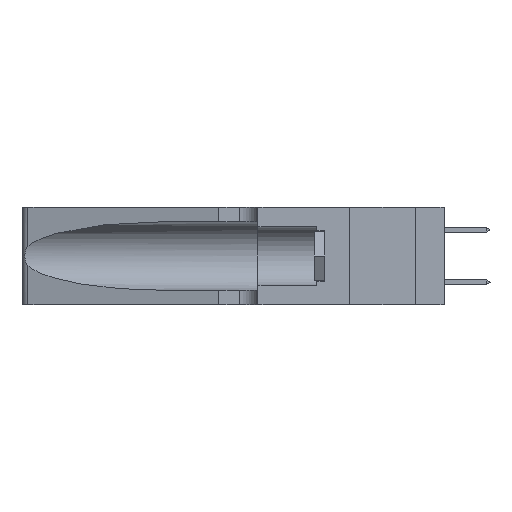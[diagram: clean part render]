
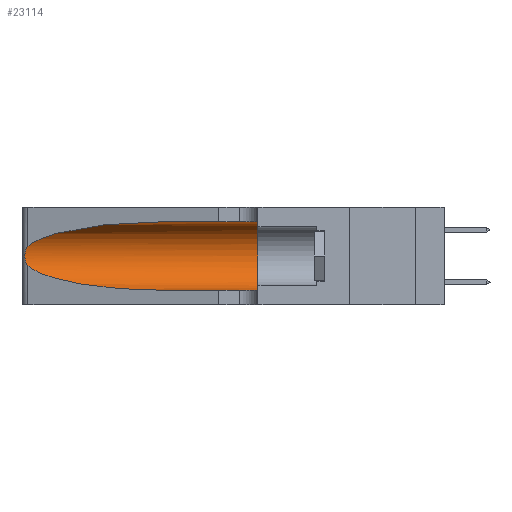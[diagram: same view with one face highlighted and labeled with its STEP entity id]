
A CAD part, left-side view. The second image highlights one B-rep face of the part: STEP entity #23114.
In plain terms, the highlighted cylindrical face has radius 3.308 mm (diameter 6.617 mm), a partial arc.
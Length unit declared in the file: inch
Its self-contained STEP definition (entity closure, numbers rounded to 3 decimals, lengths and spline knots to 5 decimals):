
#323 = CARTESIAN_POINT ( 'NONE',  ( 0.1305, 0.35, 0.31525 ) ) ;
#590 = DIRECTION ( 'NONE',  ( 0., 0., -1. ) ) ;
#2262 = CYLINDRICAL_SURFACE ( 'NONE', #6971, 0.13025 ) ;
#3616 = VERTEX_POINT ( 'NONE', #10449 ) ;
#4100 = CARTESIAN_POINT ( 'NONE',  ( 0.2373, 1.15595, 0.28018 ) ) ;
#4143 = CARTESIAN_POINT ( 'NONE',  ( 0.25487, 1.22718, 0.22369 ) ) ;
#5192 = EDGE_CURVE ( 'NONE', #3616, #29284, #23291, .T. ) ;
#5267 = CARTESIAN_POINT ( 'NONE',  ( 0.25639, 1.23186, 0.15144 ) ) ;
#6508 = VECTOR ( 'NONE', #13267, 39.37008 ) ;
#6585 = ORIENTED_EDGE ( 'NONE', *, *, #8173, .F. ) ;
#6971 = AXIS2_PLACEMENT_3D ( 'NONE', #26360, #14660, #590 ) ;
#7754 = DIRECTION ( 'NONE',  ( 0., 1., 0. ) ) ;
#8173 = EDGE_CURVE ( 'NONE', #17801, #29284, #23668, .T. ) ;
#8217 =( BOUNDED_CURVE ( )  B_SPLINE_CURVE ( 3, ( #29829, #20139, #4100, #13426 ),
 .UNSPECIFIED., .F., .T. ) 
 B_SPLINE_CURVE_WITH_KNOTS ( ( 4, 4 ),
 ( 1.5708, 2.84003 ),
 .UNSPECIFIED. ) 
 CURVE ( )  GEOMETRIC_REPRESENTATION_ITEM ( )  RATIONAL_B_SPLINE_CURVE ( ( 1., 0.87, 0.87, 1. ) ) 
 REPRESENTATION_ITEM ( '' )  );
#9820 = CARTESIAN_POINT ( 'NONE',  ( 0.26075, 1.23896, 0.178 ) ) ;
#9946 = DIRECTION ( 'NONE',  ( 0., -1., 0. ) ) ;
#10323 = CARTESIAN_POINT ( 'NONE',  ( 0.1305, 0.72297, 0.05475 ) ) ;
#10449 = CARTESIAN_POINT ( 'NONE',  ( 0.1305, 0.72297, 0.05475 ) ) ;
#10504 = EDGE_CURVE ( 'NONE', #26770, #17801, #19551, .T. ) ;
#11124 = AXIS2_PLACEMENT_3D ( 'NONE', #28640, #7754, #24060 ) ;
#12274 = CARTESIAN_POINT ( 'NONE',  ( 0.25856, 1.23593, 0.16098 ) ) ;
#12296 = CARTESIAN_POINT ( 'NONE',  ( 0.1305, 1.61858, 0.31525 ) ) ;
#12854 = EDGE_CURVE ( 'NONE', #14922, #3616, #19959, .T. ) ;
#13267 = DIRECTION ( 'NONE',  ( 0., -1., 0. ) ) ;
#13426 = CARTESIAN_POINT ( 'NONE',  ( 0.25487, 1.22718, 0.22369 ) ) ;
#14338 = CARTESIAN_POINT ( 'NONE',  ( 0.25789, 1.23486, 0.15765 ) ) ;
#14435 = CARTESIAN_POINT ( 'NONE',  ( 0.25787, 1.23484, 0.2124 ) ) ;
#14465 = VECTOR ( 'NONE', #9946, 39.37008 ) ;
#14531 = CARTESIAN_POINT ( 'NONE',  ( 0.26075, 1.23896, 0.19203 ) ) ;
#14634 = CARTESIAN_POINT ( 'NONE',  ( 0.25487, 1.22718, 0.14631 ) ) ;
#14660 = DIRECTION ( 'NONE',  ( 0., -1., 0. ) ) ;
#14922 = VERTEX_POINT ( 'NONE', #20444 ) ;
#15212 = EDGE_CURVE ( 'NONE', #28471, #14922, #27092, .T. ) ;
#15296 = ORIENTED_EDGE ( 'NONE', *, *, #5192, .T. ) ;
#16530 = CARTESIAN_POINT ( 'NONE',  ( 0.1305, 0.72297, 0.31525 ) ) ;
#16789 = CARTESIAN_POINT ( 'NONE',  ( 0.26017, 1.23833, 0.17102 ) ) ;
#17176 = CARTESIAN_POINT ( 'NONE',  ( 0.25487, 1.22718, 0.14631 ) ) ;
#17801 = VERTEX_POINT ( 'NONE', #323 ) ;
#18909 = CARTESIAN_POINT ( 'NONE',  ( 0.25854, 1.2359, 0.20912 ) ) ;
#18991 = EDGE_CURVE ( 'NONE', #26770, #28471, #8217, .T. ) ;
#19551 = LINE ( 'NONE', #12296, #14465 ) ;
#19597 = CARTESIAN_POINT ( 'NONE',  ( 0.2373, 1.15595, 0.08982 ) ) ;
#19959 =( BOUNDED_CURVE ( )  B_SPLINE_CURVE ( 3, ( #17176, #19597, #21950, #10323 ),
 .UNSPECIFIED., .F., .F. ) 
 B_SPLINE_CURVE_WITH_KNOTS ( ( 4, 4 ),
 ( 3.44316, 4.71239 ),
 .UNSPECIFIED. ) 
 CURVE ( )  GEOMETRIC_REPRESENTATION_ITEM ( )  RATIONAL_B_SPLINE_CURVE ( ( 1., 0.87, 0.87, 1. ) ) 
 REPRESENTATION_ITEM ( '' )  );
#20139 = CARTESIAN_POINT ( 'NONE',  ( 0.18966, 0.96281, 0.31525 ) ) ;
#20229 = ORIENTED_EDGE ( 'NONE', *, *, #18991, .T. ) ;
#20295 = CARTESIAN_POINT ( 'NONE',  ( 0.1305, 1.61858, 0.05475 ) ) ;
#20444 = CARTESIAN_POINT ( 'NONE',  ( 0.25487, 1.22718, 0.14631 ) ) ;
#20491 = CARTESIAN_POINT ( 'NONE',  ( 0.1305, 0.35, 0.05475 ) ) ;
#21332 = CARTESIAN_POINT ( 'NONE',  ( 0.25555, 1.22993, 0.14849 ) ) ;
#21556 = FACE_OUTER_BOUND ( 'NONE', #22738, .T. ) ;
#21950 = CARTESIAN_POINT ( 'NONE',  ( 0.18966, 0.96281, 0.05475 ) ) ;
#22738 = EDGE_LOOP ( 'NONE', ( #20229, #25812, #25232, #15296, #6585, #25080 ) ) ;
#23114 = ADVANCED_FACE ( 'NONE', ( #21556 ), #2262, .F. ) ;
#23291 = LINE ( 'NONE', #20295, #6508 ) ;
#23668 = CIRCLE ( 'NONE', #11124, 0.13025 ) ;
#23702 = CARTESIAN_POINT ( 'NONE',  ( 0.25639, 1.23184, 0.21858 ) ) ;
#24060 = DIRECTION ( 'NONE',  ( 0., 0., 1. ) ) ;
#25080 = ORIENTED_EDGE ( 'NONE', *, *, #10504, .F. ) ;
#25232 = ORIENTED_EDGE ( 'NONE', *, *, #12854, .T. ) ;
#25812 = ORIENTED_EDGE ( 'NONE', *, *, #15212, .T. ) ;
#26360 = CARTESIAN_POINT ( 'NONE',  ( 0.1305, 1.61858, 0.185 ) ) ;
#26770 = VERTEX_POINT ( 'NONE', #16530 ) ;
#27092 = B_SPLINE_CURVE_WITH_KNOTS ( 'NONE', 3,
 ( #28379, #28272, #23702, #14435, #18909, #28481, #14531, #9820, #16789, #12274, #14338, #5267, #21332, #14634 ),
 .UNSPECIFIED., .F., .F.,
 ( 4, 2, 2, 2, 2, 2, 4 ),
 ( 0., 0.00027, 0.00053, 0.00107, 0.0016, 0.00187, 0.00214 ),
 .UNSPECIFIED. ) ;
#28272 = CARTESIAN_POINT ( 'NONE',  ( 0.25555, 1.22994, 0.2215 ) ) ;
#28379 = CARTESIAN_POINT ( 'NONE',  ( 0.25487, 1.22718, 0.22369 ) ) ;
#28471 = VERTEX_POINT ( 'NONE', #4143 ) ;
#28481 = CARTESIAN_POINT ( 'NONE',  ( 0.26018, 1.23835, 0.19895 ) ) ;
#28640 = CARTESIAN_POINT ( 'NONE',  ( 0.1305, 0.35, 0.185 ) ) ;
#29284 = VERTEX_POINT ( 'NONE', #20491 ) ;
#29829 = CARTESIAN_POINT ( 'NONE',  ( 0.1305, 0.72297, 0.31525 ) ) ;
